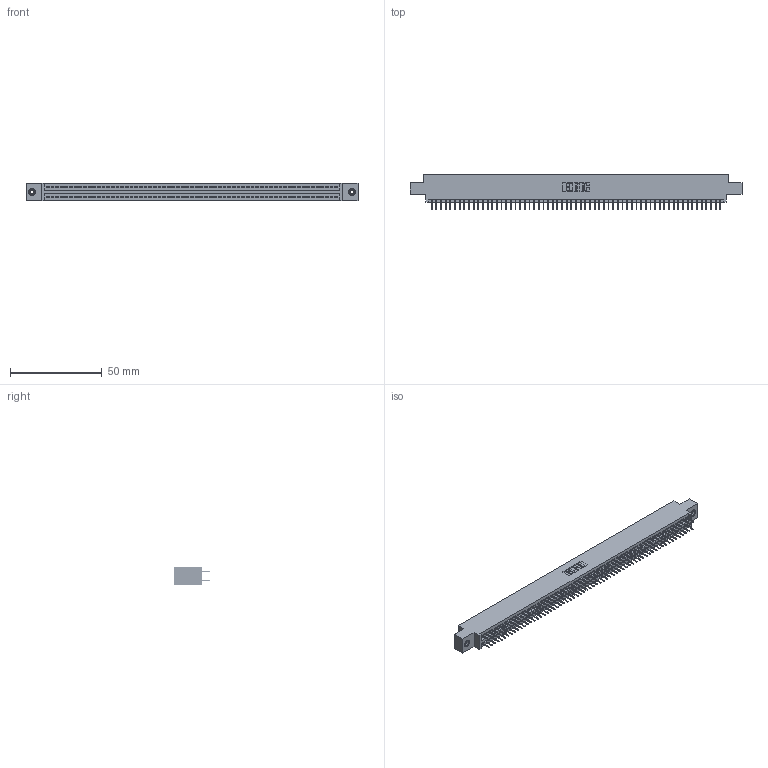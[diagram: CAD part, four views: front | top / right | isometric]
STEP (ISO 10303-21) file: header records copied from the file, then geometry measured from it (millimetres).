
FILE_DESCRIPTION (( 'STEP AP203' ), '1' );
FILE_NAME ('345-126-524-808.STEP', '2018-10-19T13:35:14', ( '' ), ( '' ), 'SwSTEP 2.0', 'SolidWorks 2016', '' );
FILE_SCHEMA (( 'CONFIG_CONTROL_DESIGN' ));
Length unit declared in the file: inch
Products named in the file (4): 345-292-001_345-293-124; 345-126-524-808; 345-250-001_345-250-003-102; 345 Part_0.170 Offset - 0.156 Dia-TI
Assembly tree (129 placements, depth 2):
  345-126-524-808
    345 Part_0.170 Offset - 0.156 Dia-TI
    345-292-001_345-293-124  x126
    345-250-001_345-250-003-102  x2
Bounding box: 181.23 x 19.35 x 9.4 mm (x, y, z)
Volume: 17489.1 mm3; surface area: 25912.1 mm2
Topology: 129 solids, 129 shells, 6994 faces, 19767 edges, 12666 vertices
Faces by surface type: plane 5030, cylinder 1948, cone 12, torus 4
Entity records: 47996 total; most frequent: CARTESIAN_POINT 8007, ORIENTED_EDGE 7934, DIRECTION 7061, EDGE_CURVE 3967, LINE 3567, VECTOR 3567, VERTEX_POINT 2636, AXIS2_PLACEMENT_3D 1747
